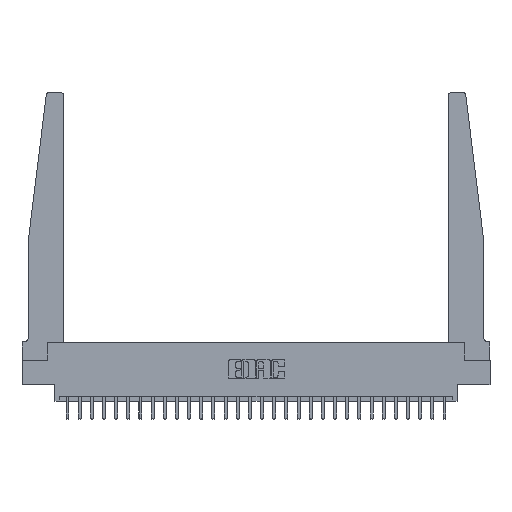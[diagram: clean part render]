
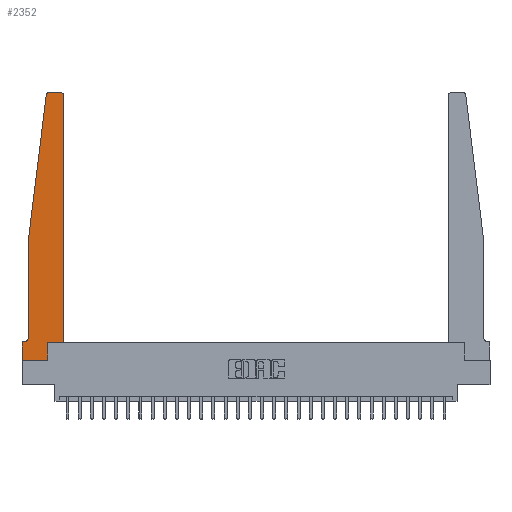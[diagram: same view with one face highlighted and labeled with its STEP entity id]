
A CAD part, top view. The second image highlights one B-rep face of the part: STEP entity #2352.
In plain terms, the highlighted planar face has unit normal (0, 0, 1).
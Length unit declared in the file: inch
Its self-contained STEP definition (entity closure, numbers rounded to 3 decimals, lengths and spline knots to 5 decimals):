
#42 = VERTEX_POINT ( 'NONE', #10809 ) ;
#436 = CARTESIAN_POINT ( 'NONE',  ( 0.25, 2.75, 0.37 ) ) ;
#780 = ORIENTED_EDGE ( 'NONE', *, *, #9948, .T. ) ;
#1363 = LINE ( 'NONE', #18400, #17630 ) ;
#1754 = CIRCLE ( 'NONE', #24626, 0.03 ) ;
#1827 = ORIENTED_EDGE ( 'NONE', *, *, #11871, .T. ) ;
#1864 = CARTESIAN_POINT ( 'NONE',  ( 0., 0., 0.37 ) ) ;
#1992 = CARTESIAN_POINT ( 'NONE',  ( 0.065, 0.2375, 0.37 ) ) ;
#2352 = ADVANCED_FACE ( 'NONE', ( #4251 ), #16754, .T. ) ;
#2522 = DIRECTION ( 'NONE',  ( 0., 0., -1. ) ) ;
#2629 = VERTEX_POINT ( 'NONE', #25936 ) ;
#3170 = AXIS2_PLACEMENT_3D ( 'NONE', #5409, #20150, #7562 ) ;
#3362 = ORIENTED_EDGE ( 'NONE', *, *, #5270, .T. ) ;
#3562 = ORIENTED_EDGE ( 'NONE', *, *, #22498, .T. ) ;
#3580 = DIRECTION ( 'NONE',  ( 1., 0., 0. ) ) ;
#3885 = VERTEX_POINT ( 'NONE', #4874 ) ;
#4068 = LINE ( 'NONE', #17665, #25731 ) ;
#4251 = FACE_OUTER_BOUND ( 'NONE', #12102, .T. ) ;
#4326 = VERTEX_POINT ( 'NONE', #1992 ) ;
#4674 = VECTOR ( 'NONE', #18352, 39.37008 ) ;
#4874 = CARTESIAN_POINT ( 'NONE',  ( 0., 0.1875, 0.37 ) ) ;
#4898 = VECTOR ( 'NONE', #10623, 39.37008 ) ;
#4932 = DIRECTION ( 'NONE',  ( -1., 0., 0. ) ) ;
#4977 = VERTEX_POINT ( 'NONE', #11177 ) ;
#5270 = EDGE_CURVE ( 'NONE', #2629, #4326, #23659, .T. ) ;
#5409 = CARTESIAN_POINT ( 'NONE',  ( 0.395, 2.72, 0.37 ) ) ;
#6249 = ORIENTED_EDGE ( 'NONE', *, *, #17511, .T. ) ;
#7562 = DIRECTION ( 'NONE',  ( 1., 0., 0. ) ) ;
#7585 = VECTOR ( 'NONE', #10131, 39.37008 ) ;
#8004 = LINE ( 'NONE', #27265, #23429 ) ;
#8086 = CARTESIAN_POINT ( 'NONE',  ( 0.015, 0.1875, 0.37 ) ) ;
#8242 = AXIS2_PLACEMENT_3D ( 'NONE', #18847, #22982, #10487 ) ;
#8252 = EDGE_CURVE ( 'NONE', #15908, #42, #1754, .T. ) ;
#8362 = ORIENTED_EDGE ( 'NONE', *, *, #25274, .T. ) ;
#8552 = DIRECTION ( 'NONE',  ( -1., 0., 0. ) ) ;
#8669 = CARTESIAN_POINT ( 'NONE',  ( 0.27653, 2.72, 0.37 ) ) ;
#9113 = EDGE_CURVE ( 'NONE', #17200, #19898, #4068, .T. ) ;
#9206 = ORIENTED_EDGE ( 'NONE', *, *, #9113, .T. ) ;
#9935 = LINE ( 'NONE', #23112, #4898 ) ;
#9948 = EDGE_CURVE ( 'NONE', #25516, #4977, #18602, .T. ) ;
#10049 = EDGE_CURVE ( 'NONE', #13536, #17200, #10367, .T. ) ;
#10131 = DIRECTION ( 'NONE',  ( 0., -1., 0. ) ) ;
#10367 = LINE ( 'NONE', #26551, #4674 ) ;
#10388 = EDGE_CURVE ( 'NONE', #17422, #3885, #8004, .T. ) ;
#10487 = DIRECTION ( 'NONE',  ( 1., 0., 0. ) ) ;
#10623 = DIRECTION ( 'NONE',  ( 0., 1., 0. ) ) ;
#10699 = CIRCLE ( 'NONE', #19165, 0.05 ) ;
#10803 = EDGE_CURVE ( 'NONE', #19412, #13536, #1363, .T. ) ;
#10809 = CARTESIAN_POINT ( 'NONE',  ( 0.24675, 2.72367, 0.37 ) ) ;
#10832 = DIRECTION ( 'NONE',  ( 1., 0., 0. ) ) ;
#10992 = LINE ( 'NONE', #1864, #21441 ) ;
#11177 = CARTESIAN_POINT ( 'NONE',  ( 0.395, 2.75, 0.37 ) ) ;
#11871 = EDGE_CURVE ( 'NONE', #42, #2629, #26612, .T. ) ;
#11981 = CARTESIAN_POINT ( 'NONE',  ( 0.2605, 0., 0.37 ) ) ;
#12077 = EDGE_CURVE ( 'NONE', #3885, #19412, #10992, .T. ) ;
#12102 = EDGE_LOOP ( 'NONE', ( #8362, #23994, #1827, #3362, #3562, #17214, #19450, #13824, #21894, #9206, #6249, #780 ) ) ;
#12288 = LINE ( 'NONE', #436, #17182 ) ;
#13536 = VERTEX_POINT ( 'NONE', #11981 ) ;
#13806 = CARTESIAN_POINT ( 'NONE',  ( 0.065, 1.25, 0.37 ) ) ;
#13824 = ORIENTED_EDGE ( 'NONE', *, *, #10803, .T. ) ;
#15236 = CARTESIAN_POINT ( 'NONE',  ( 0.015, 0.2375, 0.37 ) ) ;
#15908 = VERTEX_POINT ( 'NONE', #19799 ) ;
#16754 = PLANE ( 'NONE',  #8242 ) ;
#17182 = VECTOR ( 'NONE', #4932, 39.37008 ) ;
#17200 = VERTEX_POINT ( 'NONE', #19616 ) ;
#17214 = ORIENTED_EDGE ( 'NONE', *, *, #10388, .T. ) ;
#17323 = DIRECTION ( 'NONE',  ( -1., 0., 0. ) ) ;
#17422 = VERTEX_POINT ( 'NONE', #8086 ) ;
#17511 = EDGE_CURVE ( 'NONE', #19898, #25516, #9935, .T. ) ;
#17630 = VECTOR ( 'NONE', #3580, 39.37008 ) ;
#17665 = CARTESIAN_POINT ( 'NONE',  ( 0.425, 0.18, 0.37 ) ) ;
#18352 = DIRECTION ( 'NONE',  ( 0., 1., 0. ) ) ;
#18400 = CARTESIAN_POINT ( 'NONE',  ( 0., 0., 0.37 ) ) ;
#18439 = CARTESIAN_POINT ( 'NONE',  ( 0.425, 2.72, 0.37 ) ) ;
#18602 = CIRCLE ( 'NONE', #3170, 0.03 ) ;
#18847 = CARTESIAN_POINT ( 'NONE',  ( 0., 0.1875, 0.37 ) ) ;
#19165 = AXIS2_PLACEMENT_3D ( 'NONE', #15236, #2522, #17323 ) ;
#19238 = CARTESIAN_POINT ( 'NONE',  ( 0., 0., 0.37 ) ) ;
#19412 = VERTEX_POINT ( 'NONE', #19238 ) ;
#19450 = ORIENTED_EDGE ( 'NONE', *, *, #12077, .T. ) ;
#19616 = CARTESIAN_POINT ( 'NONE',  ( 0.2605, 0.18, 0.37 ) ) ;
#19764 = DIRECTION ( 'NONE',  ( 1., 0., 0. ) ) ;
#19799 = CARTESIAN_POINT ( 'NONE',  ( 0.27653, 2.75, 0.37 ) ) ;
#19898 = VERTEX_POINT ( 'NONE', #24888 ) ;
#19989 = DIRECTION ( 'NONE',  ( -0.122, -0.992, 0. ) ) ;
#20150 = DIRECTION ( 'NONE',  ( 0., 0., 1. ) ) ;
#20473 = VECTOR ( 'NONE', #19989, 39.37008 ) ;
#20853 = DIRECTION ( 'NONE',  ( 0., -1., 0. ) ) ;
#21441 = VECTOR ( 'NONE', #20853, 39.37008 ) ;
#21894 = ORIENTED_EDGE ( 'NONE', *, *, #10049, .T. ) ;
#22498 = EDGE_CURVE ( 'NONE', #4326, #17422, #10699, .T. ) ;
#22982 = DIRECTION ( 'NONE',  ( 0., 0., 1. ) ) ;
#23112 = CARTESIAN_POINT ( 'NONE',  ( 0.425, 0.18, 0.37 ) ) ;
#23329 = DIRECTION ( 'NONE',  ( 0., 0., 1. ) ) ;
#23429 = VECTOR ( 'NONE', #8552, 39.37008 ) ;
#23659 = LINE ( 'NONE', #24732, #7585 ) ;
#23994 = ORIENTED_EDGE ( 'NONE', *, *, #8252, .T. ) ;
#24626 = AXIS2_PLACEMENT_3D ( 'NONE', #8669, #23329, #10832 ) ;
#24732 = CARTESIAN_POINT ( 'NONE',  ( 0.065, 1.25, 0.37 ) ) ;
#24888 = CARTESIAN_POINT ( 'NONE',  ( 0.425, 0.18, 0.37 ) ) ;
#25274 = EDGE_CURVE ( 'NONE', #4977, #15908, #12288, .T. ) ;
#25516 = VERTEX_POINT ( 'NONE', #18439 ) ;
#25731 = VECTOR ( 'NONE', #19764, 39.37008 ) ;
#25936 = CARTESIAN_POINT ( 'NONE',  ( 0.065, 1.25, 0.37 ) ) ;
#26551 = CARTESIAN_POINT ( 'NONE',  ( 0.2605, 0.18, 0.37 ) ) ;
#26612 = LINE ( 'NONE', #13806, #20473 ) ;
#27265 = CARTESIAN_POINT ( 'NONE',  ( 0.065, 0.1875, 0.37 ) ) ;
